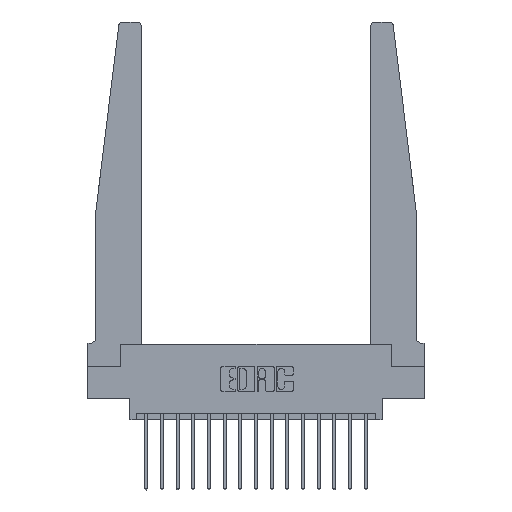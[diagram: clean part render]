
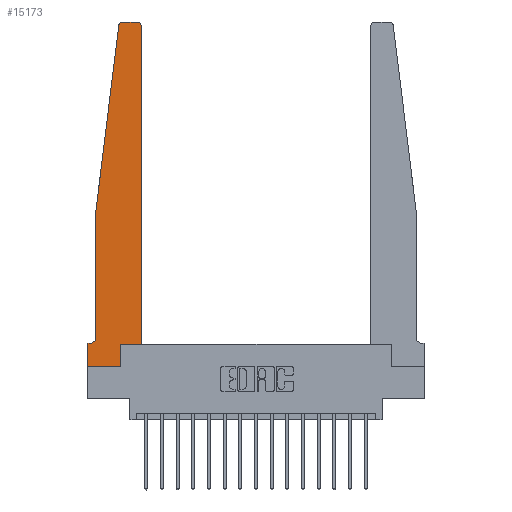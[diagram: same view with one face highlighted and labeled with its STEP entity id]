
A CAD part, top view. The second image highlights one B-rep face of the part: STEP entity #15173.
In plain terms, the highlighted planar face has unit normal (0, 0, 1).
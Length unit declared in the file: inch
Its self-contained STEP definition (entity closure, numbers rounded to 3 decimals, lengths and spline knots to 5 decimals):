
#37 = ORIENTED_EDGE ( 'NONE', *, *, #12282, .T. ) ;
#151 = CARTESIAN_POINT ( 'NONE',  ( 0.425, 0.18, 0.37 ) ) ;
#551 = CARTESIAN_POINT ( 'NONE',  ( 0.015, 0.1875, 0.37 ) ) ;
#693 = CARTESIAN_POINT ( 'NONE',  ( 0.065, 0.1875, 0.37 ) ) ;
#766 = ORIENTED_EDGE ( 'NONE', *, *, #13554, .T. ) ;
#800 = CARTESIAN_POINT ( 'NONE',  ( 0.065, 1.25, 0.37 ) ) ;
#1538 = ORIENTED_EDGE ( 'NONE', *, *, #12921, .T. ) ;
#1647 = ORIENTED_EDGE ( 'NONE', *, *, #3427, .T. ) ;
#1857 = CARTESIAN_POINT ( 'NONE',  ( 0.065, 0.2375, 0.37 ) ) ;
#1998 = EDGE_CURVE ( 'NONE', #13944, #7214, #12873, .T. ) ;
#2037 = CARTESIAN_POINT ( 'NONE',  ( 0.25, 2.75, 0.37 ) ) ;
#2328 = VECTOR ( 'NONE', #5632, 39.37008 ) ;
#2650 = VERTEX_POINT ( 'NONE', #11083 ) ;
#2724 = DIRECTION ( 'NONE',  ( 0., 0., -1. ) ) ;
#2808 = DIRECTION ( 'NONE',  ( 0., 1., 0. ) ) ;
#3127 = VERTEX_POINT ( 'NONE', #551 ) ;
#3414 = VERTEX_POINT ( 'NONE', #5551 ) ;
#3427 = EDGE_CURVE ( 'NONE', #11711, #3127, #4199, .T. ) ;
#3457 = VERTEX_POINT ( 'NONE', #12712 ) ;
#3661 = LINE ( 'NONE', #11581, #6980 ) ;
#3942 = DIRECTION ( 'NONE',  ( 0., 0., 1. ) ) ;
#4131 = CARTESIAN_POINT ( 'NONE',  ( 0.425, 0.18, 0.37 ) ) ;
#4199 = CIRCLE ( 'NONE', #7978, 0.05 ) ;
#4324 = EDGE_CURVE ( 'NONE', #3127, #4573, #16307, .T. ) ;
#4573 = VERTEX_POINT ( 'NONE', #8283 ) ;
#4934 = DIRECTION ( 'NONE',  ( 1., 0., 0. ) ) ;
#5431 = VERTEX_POINT ( 'NONE', #15793 ) ;
#5488 = CARTESIAN_POINT ( 'NONE',  ( 0.395, 2.72, 0.37 ) ) ;
#5504 = VECTOR ( 'NONE', #10635, 39.37008 ) ;
#5551 = CARTESIAN_POINT ( 'NONE',  ( 0., 0., 0.37 ) ) ;
#5632 = DIRECTION ( 'NONE',  ( 0., 1., 0. ) ) ;
#5707 = EDGE_CURVE ( 'NONE', #9606, #5431, #7219, .T. ) ;
#5853 = VECTOR ( 'NONE', #2808, 39.37008 ) ;
#6114 = LINE ( 'NONE', #4131, #2328 ) ;
#6417 = VECTOR ( 'NONE', #4934, 39.37008 ) ;
#6877 = DIRECTION ( 'NONE',  ( 1., 0., 0. ) ) ;
#6980 = VECTOR ( 'NONE', #15898, 39.37008 ) ;
#7214 = VERTEX_POINT ( 'NONE', #18157 ) ;
#7219 = LINE ( 'NONE', #800, #8093 ) ;
#7439 = CARTESIAN_POINT ( 'NONE',  ( 0.425, 2.72, 0.37 ) ) ;
#7978 = AXIS2_PLACEMENT_3D ( 'NONE', #11232, #2724, #12650 ) ;
#8093 = VECTOR ( 'NONE', #12164, 39.37008 ) ;
#8280 = ORIENTED_EDGE ( 'NONE', *, *, #15028, .T. ) ;
#8283 = CARTESIAN_POINT ( 'NONE',  ( 0., 0.1875, 0.37 ) ) ;
#8464 = CARTESIAN_POINT ( 'NONE',  ( 0., 0.1875, 0.37 ) ) ;
#8504 = VERTEX_POINT ( 'NONE', #11521 ) ;
#8581 = LINE ( 'NONE', #13142, #15645 ) ;
#9131 = CARTESIAN_POINT ( 'NONE',  ( 0.2605, 0.18, 0.37 ) ) ;
#9606 = VERTEX_POINT ( 'NONE', #9688 ) ;
#9656 = ORIENTED_EDGE ( 'NONE', *, *, #5707, .T. ) ;
#9688 = CARTESIAN_POINT ( 'NONE',  ( 0.24675, 2.72367, 0.37 ) ) ;
#9890 = DIRECTION ( 'NONE',  ( 1., 0., 0. ) ) ;
#9893 = CARTESIAN_POINT ( 'NONE',  ( 0.2605, 0.18, 0.37 ) ) ;
#9928 = ORIENTED_EDGE ( 'NONE', *, *, #16806, .T. ) ;
#10005 = VECTOR ( 'NONE', #10111, 39.37008 ) ;
#10111 = DIRECTION ( 'NONE',  ( 1., 0., 0. ) ) ;
#10197 = LINE ( 'NONE', #10324, #6417 ) ;
#10324 = CARTESIAN_POINT ( 'NONE',  ( 0., 0., 0.37 ) ) ;
#10635 = DIRECTION ( 'NONE',  ( -1., 0., 0. ) ) ;
#10770 = FACE_OUTER_BOUND ( 'NONE', #12586, .T. ) ;
#10822 = LINE ( 'NONE', #2037, #18330 ) ;
#11083 = CARTESIAN_POINT ( 'NONE',  ( 0.2605, 0., 0.37 ) ) ;
#11232 = CARTESIAN_POINT ( 'NONE',  ( 0.015, 0.2375, 0.37 ) ) ;
#11521 = CARTESIAN_POINT ( 'NONE',  ( 0.27653, 2.75, 0.37 ) ) ;
#11581 = CARTESIAN_POINT ( 'NONE',  ( 0.065, 1.25, 0.37 ) ) ;
#11711 = VERTEX_POINT ( 'NONE', #1857 ) ;
#11963 = DIRECTION ( 'NONE',  ( -1., 0., 0. ) ) ;
#12031 = ORIENTED_EDGE ( 'NONE', *, *, #15157, .T. ) ;
#12164 = DIRECTION ( 'NONE',  ( -0.122, -0.992, 0. ) ) ;
#12282 = EDGE_CURVE ( 'NONE', #15480, #3457, #17934, .T. ) ;
#12423 = ORIENTED_EDGE ( 'NONE', *, *, #1998, .T. ) ;
#12427 = CARTESIAN_POINT ( 'NONE',  ( 0.27653, 2.72, 0.37 ) ) ;
#12586 = EDGE_LOOP ( 'NONE', ( #766, #8280, #9656, #16765, #1647, #17618, #16165, #1538, #9928, #37, #12031, #12423 ) ) ;
#12594 = AXIS2_PLACEMENT_3D ( 'NONE', #5488, #15350, #6877 ) ;
#12650 = DIRECTION ( 'NONE',  ( -1., 0., 0. ) ) ;
#12712 = CARTESIAN_POINT ( 'NONE',  ( 0.425, 0.18, 0.37 ) ) ;
#12873 = CIRCLE ( 'NONE', #12594, 0.03 ) ;
#12921 = EDGE_CURVE ( 'NONE', #3414, #2650, #10197, .T. ) ;
#13142 = CARTESIAN_POINT ( 'NONE',  ( 0., 0., 0.37 ) ) ;
#13554 = EDGE_CURVE ( 'NONE', #7214, #8504, #10822, .T. ) ;
#13812 = DIRECTION ( 'NONE',  ( 1., 0., 0. ) ) ;
#13846 = CIRCLE ( 'NONE', #16949, 0.03 ) ;
#13944 = VERTEX_POINT ( 'NONE', #7439 ) ;
#14558 = DIRECTION ( 'NONE',  ( 0., -1., 0. ) ) ;
#14683 = AXIS2_PLACEMENT_3D ( 'NONE', #8464, #18332, #9890 ) ;
#14738 = EDGE_CURVE ( 'NONE', #4573, #3414, #8581, .T. ) ;
#15028 = EDGE_CURVE ( 'NONE', #8504, #9606, #13846, .T. ) ;
#15157 = EDGE_CURVE ( 'NONE', #3457, #13944, #6114, .T. ) ;
#15173 = ADVANCED_FACE ( 'NONE', ( #10770 ), #16911, .T. ) ;
#15350 = DIRECTION ( 'NONE',  ( 0., 0., 1. ) ) ;
#15480 = VERTEX_POINT ( 'NONE', #9131 ) ;
#15645 = VECTOR ( 'NONE', #14558, 39.37008 ) ;
#15793 = CARTESIAN_POINT ( 'NONE',  ( 0.065, 1.25, 0.37 ) ) ;
#15898 = DIRECTION ( 'NONE',  ( 0., -1., 0. ) ) ;
#16165 = ORIENTED_EDGE ( 'NONE', *, *, #14738, .T. ) ;
#16307 = LINE ( 'NONE', #693, #5504 ) ;
#16765 = ORIENTED_EDGE ( 'NONE', *, *, #18355, .T. ) ;
#16806 = EDGE_CURVE ( 'NONE', #2650, #15480, #17118, .T. ) ;
#16911 = PLANE ( 'NONE',  #14683 ) ;
#16949 = AXIS2_PLACEMENT_3D ( 'NONE', #12427, #3942, #13812 ) ;
#17118 = LINE ( 'NONE', #9893, #5853 ) ;
#17618 = ORIENTED_EDGE ( 'NONE', *, *, #4324, .T. ) ;
#17934 = LINE ( 'NONE', #151, #10005 ) ;
#18157 = CARTESIAN_POINT ( 'NONE',  ( 0.395, 2.75, 0.37 ) ) ;
#18330 = VECTOR ( 'NONE', #11963, 39.37008 ) ;
#18332 = DIRECTION ( 'NONE',  ( 0., 0., 1. ) ) ;
#18355 = EDGE_CURVE ( 'NONE', #5431, #11711, #3661, .T. ) ;
